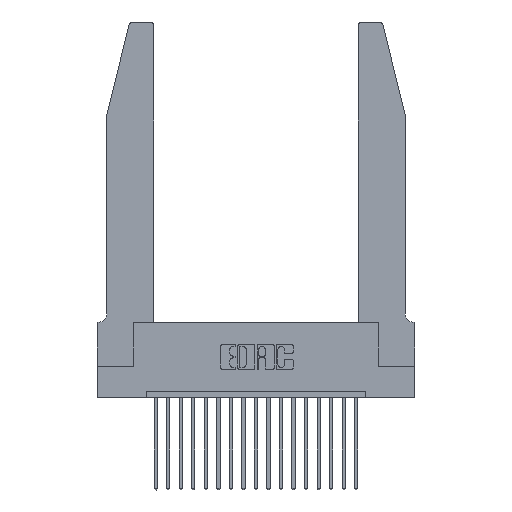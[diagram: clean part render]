
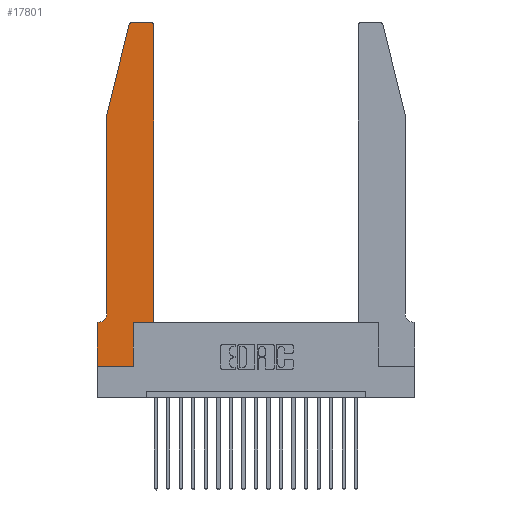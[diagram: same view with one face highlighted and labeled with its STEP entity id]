
A CAD part, top view. The second image highlights one B-rep face of the part: STEP entity #17801.
In plain terms, the highlighted planar face has unit normal (0, 0, 1).
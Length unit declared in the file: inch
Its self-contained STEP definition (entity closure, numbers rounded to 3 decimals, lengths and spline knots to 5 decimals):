
#300 = DIRECTION ( 'NONE',  ( 0., 0., 1. ) ) ;
#372 = LINE ( 'NONE', #17587, #8959 ) ;
#410 = ORIENTED_EDGE ( 'NONE', *, *, #18034, .T. ) ;
#476 = CARTESIAN_POINT ( 'NONE',  ( 0.4205, 2.72, 0.37 ) ) ;
#779 = EDGE_LOOP ( 'NONE', ( #15241, #8603, #1730, #7534, #15446, #6592, #15031, #13399, #410, #2925, #9504, #1543 ) ) ;
#1155 = LINE ( 'NONE', #7694, #9988 ) ;
#1359 = CARTESIAN_POINT ( 'NONE',  ( 0., 0., 0.37 ) ) ;
#1543 = ORIENTED_EDGE ( 'NONE', *, *, #10673, .T. ) ;
#1730 = ORIENTED_EDGE ( 'NONE', *, *, #17444, .T. ) ;
#1799 = CARTESIAN_POINT ( 'NONE',  ( 0.2865, 0.35, 0.37 ) ) ;
#1943 = VECTOR ( 'NONE', #13198, 39.37008 ) ;
#2176 = DIRECTION ( 'NONE',  ( 0., 0., 1. ) ) ;
#2318 = CIRCLE ( 'NONE', #12109, 0.07 ) ;
#2652 = DIRECTION ( 'NONE',  ( 0., 0., -1. ) ) ;
#2925 = ORIENTED_EDGE ( 'NONE', *, *, #18845, .T. ) ;
#3537 = EDGE_CURVE ( 'NONE', #3965, #9787, #5035, .T. ) ;
#3965 = VERTEX_POINT ( 'NONE', #20004 ) ;
#4187 = CARTESIAN_POINT ( 'NONE',  ( 0.25487, 2.72718, 0.37 ) ) ;
#4236 = EDGE_CURVE ( 'NONE', #17836, #6448, #16221, .T. ) ;
#5035 = LINE ( 'NONE', #7180, #8809 ) ;
#5171 = CARTESIAN_POINT ( 'NONE',  ( 0.284, 2.75, 0.37 ) ) ;
#5280 = VERTEX_POINT ( 'NONE', #10457 ) ;
#5284 = LINE ( 'NONE', #10430, #18153 ) ;
#5408 = VERTEX_POINT ( 'NONE', #15815 ) ;
#5423 = CARTESIAN_POINT ( 'NONE',  ( 0.2865, 0., 0.37 ) ) ;
#5793 = DIRECTION ( 'NONE',  ( 0., 1., 0. ) ) ;
#6064 = AXIS2_PLACEMENT_3D ( 'NONE', #19640, #300, #8424 ) ;
#6448 = VERTEX_POINT ( 'NONE', #14969 ) ;
#6592 = ORIENTED_EDGE ( 'NONE', *, *, #4236, .T. ) ;
#7118 = AXIS2_PLACEMENT_3D ( 'NONE', #9224, #20817, #15715 ) ;
#7180 = CARTESIAN_POINT ( 'NONE',  ( 0.2605, 2.75, 0.37 ) ) ;
#7534 = ORIENTED_EDGE ( 'NONE', *, *, #9323, .T. ) ;
#7632 = VECTOR ( 'NONE', #10929, 39.37008 ) ;
#7694 = CARTESIAN_POINT ( 'NONE',  ( 0.4505, 0.35, 0.37 ) ) ;
#7731 = CARTESIAN_POINT ( 'NONE',  ( 0.0755, 0.35, 0.37 ) ) ;
#7743 = CARTESIAN_POINT ( 'NONE',  ( 0.0055, 0.35, 0.37 ) ) ;
#7871 = VECTOR ( 'NONE', #5793, 39.37008 ) ;
#8424 = DIRECTION ( 'NONE',  ( 1., 0., 0. ) ) ;
#8462 = DIRECTION ( 'NONE',  ( 1., 0., 0. ) ) ;
#8603 = ORIENTED_EDGE ( 'NONE', *, *, #20331, .T. ) ;
#8809 = VECTOR ( 'NONE', #10311, 39.37008 ) ;
#8959 = VECTOR ( 'NONE', #19069, 39.37008 ) ;
#9165 = CIRCLE ( 'NONE', #6064, 0.03 ) ;
#9224 = CARTESIAN_POINT ( 'NONE',  ( 0., 0.35, 0.37 ) ) ;
#9323 = EDGE_CURVE ( 'NONE', #19559, #15995, #372, .T. ) ;
#9400 = CARTESIAN_POINT ( 'NONE',  ( 0., 0., 0.37 ) ) ;
#9426 = CARTESIAN_POINT ( 'NONE',  ( 0.0755, 2., 0.37 ) ) ;
#9504 = ORIENTED_EDGE ( 'NONE', *, *, #11775, .T. ) ;
#9787 = VERTEX_POINT ( 'NONE', #5171 ) ;
#9857 = CARTESIAN_POINT ( 'NONE',  ( 0.0755, 0.42, 0.37 ) ) ;
#9988 = VECTOR ( 'NONE', #10958, 39.37008 ) ;
#10173 = EDGE_CURVE ( 'NONE', #15998, #12892, #11420, .T. ) ;
#10311 = DIRECTION ( 'NONE',  ( -1., 0., 0. ) ) ;
#10430 = CARTESIAN_POINT ( 'NONE',  ( 0.0755, 2., 0.37 ) ) ;
#10457 = CARTESIAN_POINT ( 'NONE',  ( 0.2865, 0.35, 0.37 ) ) ;
#10673 = EDGE_CURVE ( 'NONE', #5408, #3965, #18021, .T. ) ;
#10848 = DIRECTION ( 'NONE',  ( 0., -1., 0. ) ) ;
#10929 = DIRECTION ( 'NONE',  ( -1., 0., 0. ) ) ;
#10958 = DIRECTION ( 'NONE',  ( 1., 0., 0. ) ) ;
#11420 = LINE ( 'NONE', #1359, #17274 ) ;
#11775 = EDGE_CURVE ( 'NONE', #16700, #5408, #12111, .T. ) ;
#12018 = FACE_OUTER_BOUND ( 'NONE', #779, .T. ) ;
#12109 = AXIS2_PLACEMENT_3D ( 'NONE', #13971, #2652, #13902 ) ;
#12111 = LINE ( 'NONE', #15436, #7871 ) ;
#12622 = EDGE_CURVE ( 'NONE', #15995, #17836, #2318, .T. ) ;
#12892 = VERTEX_POINT ( 'NONE', #5423 ) ;
#13198 = DIRECTION ( 'NONE',  ( 0., 1., 0. ) ) ;
#13399 = ORIENTED_EDGE ( 'NONE', *, *, #10173, .T. ) ;
#13902 = DIRECTION ( 'NONE',  ( -1., 0., 0. ) ) ;
#13971 = CARTESIAN_POINT ( 'NONE',  ( 0.0055, 0.42, 0.37 ) ) ;
#14051 = LINE ( 'NONE', #1799, #1943 ) ;
#14224 = PLANE ( 'NONE',  #7118 ) ;
#14528 = VECTOR ( 'NONE', #10848, 39.37008 ) ;
#14808 = CARTESIAN_POINT ( 'NONE',  ( 0., 0., 0.37 ) ) ;
#14969 = CARTESIAN_POINT ( 'NONE',  ( 0., 0.35, 0.37 ) ) ;
#15031 = ORIENTED_EDGE ( 'NONE', *, *, #15869, .T. ) ;
#15144 = CARTESIAN_POINT ( 'NONE',  ( 0.4505, 0.35, 0.37 ) ) ;
#15241 = ORIENTED_EDGE ( 'NONE', *, *, #3537, .T. ) ;
#15387 = AXIS2_PLACEMENT_3D ( 'NONE', #476, #2176, #8462 ) ;
#15436 = CARTESIAN_POINT ( 'NONE',  ( 0.4505, 0.35, 0.37 ) ) ;
#15446 = ORIENTED_EDGE ( 'NONE', *, *, #12622, .T. ) ;
#15715 = DIRECTION ( 'NONE',  ( 1., 0., 0. ) ) ;
#15815 = CARTESIAN_POINT ( 'NONE',  ( 0.4505, 2.72, 0.37 ) ) ;
#15869 = EDGE_CURVE ( 'NONE', #6448, #15998, #18585, .T. ) ;
#15995 = VERTEX_POINT ( 'NONE', #9857 ) ;
#15998 = VERTEX_POINT ( 'NONE', #14808 ) ;
#16221 = LINE ( 'NONE', #7731, #7632 ) ;
#16700 = VERTEX_POINT ( 'NONE', #15144 ) ;
#16739 = VERTEX_POINT ( 'NONE', #4187 ) ;
#17274 = VECTOR ( 'NONE', #17660, 39.37008 ) ;
#17444 = EDGE_CURVE ( 'NONE', #16739, #19559, #5284, .T. ) ;
#17587 = CARTESIAN_POINT ( 'NONE',  ( 0.0755, 2., 0.37 ) ) ;
#17660 = DIRECTION ( 'NONE',  ( 1., 0., 0. ) ) ;
#17801 = ADVANCED_FACE ( 'NONE', ( #12018 ), #14224, .T. ) ;
#17836 = VERTEX_POINT ( 'NONE', #7743 ) ;
#18021 = CIRCLE ( 'NONE', #15387, 0.03 ) ;
#18034 = EDGE_CURVE ( 'NONE', #12892, #5280, #14051, .T. ) ;
#18153 = VECTOR ( 'NONE', #18511, 39.37008 ) ;
#18511 = DIRECTION ( 'NONE',  ( -0.239, -0.971, 0. ) ) ;
#18585 = LINE ( 'NONE', #9400, #14528 ) ;
#18845 = EDGE_CURVE ( 'NONE', #5280, #16700, #1155, .T. ) ;
#19069 = DIRECTION ( 'NONE',  ( 0., -1., 0. ) ) ;
#19559 = VERTEX_POINT ( 'NONE', #9426 ) ;
#19640 = CARTESIAN_POINT ( 'NONE',  ( 0.284, 2.72, 0.37 ) ) ;
#20004 = CARTESIAN_POINT ( 'NONE',  ( 0.4205, 2.75, 0.37 ) ) ;
#20331 = EDGE_CURVE ( 'NONE', #9787, #16739, #9165, .T. ) ;
#20817 = DIRECTION ( 'NONE',  ( 0., 0., 1. ) ) ;
